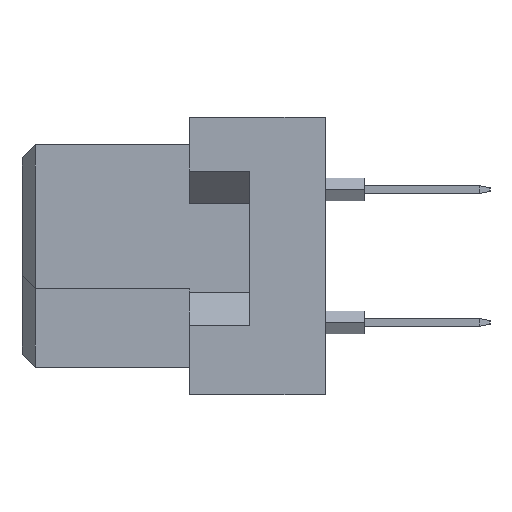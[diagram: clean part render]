
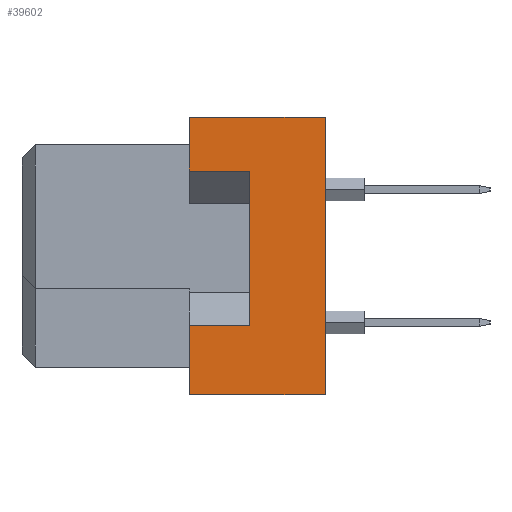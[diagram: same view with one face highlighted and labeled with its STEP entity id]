
A CAD part, left-side view. The second image highlights one B-rep face of the part: STEP entity #39602.
In plain terms, the highlighted planar face has unit normal (-1, 0, 0).
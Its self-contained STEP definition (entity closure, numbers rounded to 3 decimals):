
#132 = CARTESIAN_POINT ( 'NONE',  ( -47.5, -8.7, 3.25 ) ) ;
#857 = LINE ( 'NONE', #28592, #36057 ) ;
#1575 = EDGE_CURVE ( 'NONE', #39524, #3705, #17931, .T. ) ;
#2255 = ORIENTED_EDGE ( 'NONE', *, *, #33782, .T. ) ;
#2440 = EDGE_CURVE ( 'NONE', #22441, #16617, #27689, .T. ) ;
#2574 = CARTESIAN_POINT ( 'NONE',  ( -47.5, -6.4, 5.3 ) ) ;
#3252 = CARTESIAN_POINT ( 'NONE',  ( -47.5, -6.4, -5.3 ) ) ;
#3442 = DIRECTION ( 'NONE',  ( 0., 0., 1. ) ) ;
#3458 = ORIENTED_EDGE ( 'NONE', *, *, #2440, .F. ) ;
#3705 = VERTEX_POINT ( 'NONE', #3252 ) ;
#4395 = CARTESIAN_POINT ( 'NONE',  ( -47.5, -11.6, 5.3 ) ) ;
#5896 = EDGE_LOOP ( 'NONE', ( #2255, #21732, #19749, #10854, #18438, #39938, #35306, #3458 ) ) ;
#6464 = FACE_OUTER_BOUND ( 'NONE', #5896, .T. ) ;
#9488 = CARTESIAN_POINT ( 'NONE',  ( -47.5, -8.7, -2.65 ) ) ;
#9636 = LINE ( 'NONE', #34324, #17683 ) ;
#10051 = VERTEX_POINT ( 'NONE', #12274 ) ;
#10681 = LINE ( 'NONE', #4395, #27879 ) ;
#10854 = ORIENTED_EDGE ( 'NONE', *, *, #23553, .T. ) ;
#12206 = LINE ( 'NONE', #36272, #17906 ) ;
#12274 = CARTESIAN_POINT ( 'NONE',  ( -47.5, -6.4, 3.25 ) ) ;
#13753 = VECTOR ( 'NONE', #27238, 1000. ) ;
#14025 = VERTEX_POINT ( 'NONE', #15949 ) ;
#14910 = DIRECTION ( 'NONE',  ( 0., 1., 0. ) ) ;
#15074 = VERTEX_POINT ( 'NONE', #37686 ) ;
#15103 = EDGE_CURVE ( 'NONE', #10051, #26850, #857, .T. ) ;
#15569 = AXIS2_PLACEMENT_3D ( 'NONE', #18827, #31167, #3442 ) ;
#15949 = CARTESIAN_POINT ( 'NONE',  ( -47.5, -11.6, 5.3 ) ) ;
#16617 = VERTEX_POINT ( 'NONE', #29345 ) ;
#17243 = CARTESIAN_POINT ( 'NONE',  ( -47.5, -8.7, -2.65 ) ) ;
#17578 = DIRECTION ( 'NONE',  ( 0., 1., 0. ) ) ;
#17683 = VECTOR ( 'NONE', #28850, 1000. ) ;
#17906 = VECTOR ( 'NONE', #24153, 1000. ) ;
#17931 = LINE ( 'NONE', #21368, #13753 ) ;
#18438 = ORIENTED_EDGE ( 'NONE', *, *, #19189, .T. ) ;
#18827 = CARTESIAN_POINT ( 'NONE',  ( -47.5, -11.6, 5.3 ) ) ;
#19003 = DIRECTION ( 'NONE',  ( 0., 0., 1. ) ) ;
#19189 = EDGE_CURVE ( 'NONE', #14025, #26850, #10681, .T. ) ;
#19749 = ORIENTED_EDGE ( 'NONE', *, *, #1575, .F. ) ;
#20916 = VECTOR ( 'NONE', #14910, 1000. ) ;
#21368 = CARTESIAN_POINT ( 'NONE',  ( -47.5, -11.6, -5.3 ) ) ;
#21732 = ORIENTED_EDGE ( 'NONE', *, *, #28938, .F. ) ;
#22059 = PLANE ( 'NONE',  #15569 ) ;
#22441 = VERTEX_POINT ( 'NONE', #17243 ) ;
#23024 = DIRECTION ( 'NONE',  ( 0., 1., 0. ) ) ;
#23461 = EDGE_CURVE ( 'NONE', #16617, #10051, #33926, .T. ) ;
#23553 = EDGE_CURVE ( 'NONE', #39524, #14025, #9636, .T. ) ;
#24153 = DIRECTION ( 'NONE',  ( 0., 0., 1. ) ) ;
#24514 = VECTOR ( 'NONE', #17578, 1000. ) ;
#25751 = DIRECTION ( 'NONE',  ( 0., 0., 1. ) ) ;
#26850 = VERTEX_POINT ( 'NONE', #2574 ) ;
#27238 = DIRECTION ( 'NONE',  ( 0., 1., 0. ) ) ;
#27689 = LINE ( 'NONE', #28095, #36405 ) ;
#27879 = VECTOR ( 'NONE', #23024, 1000. ) ;
#28095 = CARTESIAN_POINT ( 'NONE',  ( -47.5, -8.7, -2.65 ) ) ;
#28592 = CARTESIAN_POINT ( 'NONE',  ( -47.5, -6.4, -5.3 ) ) ;
#28850 = DIRECTION ( 'NONE',  ( 0., 0., 1. ) ) ;
#28938 = EDGE_CURVE ( 'NONE', #3705, #15074, #12206, .T. ) ;
#29345 = CARTESIAN_POINT ( 'NONE',  ( -47.5, -8.7, 3.25 ) ) ;
#30567 = CARTESIAN_POINT ( 'NONE',  ( -47.5, -11.6, -5.3 ) ) ;
#31167 = DIRECTION ( 'NONE',  ( -1., 0., 0. ) ) ;
#33782 = EDGE_CURVE ( 'NONE', #22441, #15074, #37199, .T. ) ;
#33926 = LINE ( 'NONE', #132, #20916 ) ;
#34324 = CARTESIAN_POINT ( 'NONE',  ( -47.5, -11.6, 5.3 ) ) ;
#35306 = ORIENTED_EDGE ( 'NONE', *, *, #23461, .F. ) ;
#36057 = VECTOR ( 'NONE', #25751, 1000. ) ;
#36272 = CARTESIAN_POINT ( 'NONE',  ( -47.5, -6.4, -5.3 ) ) ;
#36405 = VECTOR ( 'NONE', #19003, 1000. ) ;
#37199 = LINE ( 'NONE', #9488, #24514 ) ;
#37686 = CARTESIAN_POINT ( 'NONE',  ( -47.5, -6.4, -2.65 ) ) ;
#39524 = VERTEX_POINT ( 'NONE', #30567 ) ;
#39602 = ADVANCED_FACE ( 'NONE', ( #6464 ), #22059, .T. ) ;
#39938 = ORIENTED_EDGE ( 'NONE', *, *, #15103, .F. ) ;
